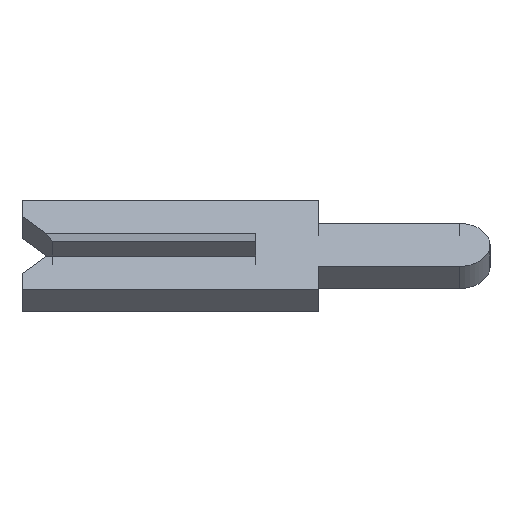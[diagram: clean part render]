
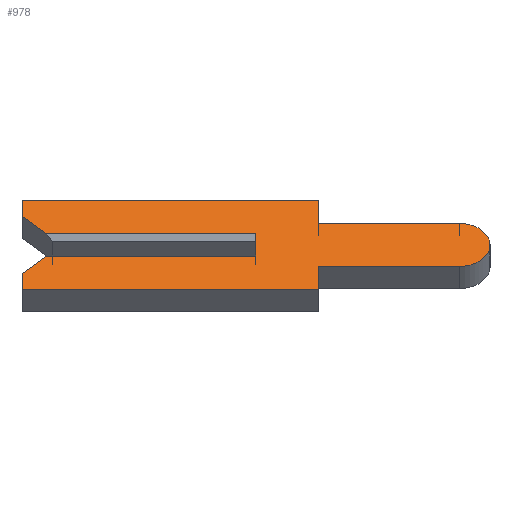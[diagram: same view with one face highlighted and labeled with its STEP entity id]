
A CAD part, left-side view. The second image highlights one B-rep face of the part: STEP entity #978.
In plain terms, the highlighted face is planar.
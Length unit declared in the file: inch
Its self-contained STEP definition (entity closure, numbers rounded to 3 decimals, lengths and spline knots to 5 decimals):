
#20 = CARTESIAN_POINT ( 'NONE',  ( -0.01, -0.04, 0.04 ) ) ;
#44 = LINE ( 'NONE', #263, #1653 ) ;
#54 = ORIENTED_EDGE ( 'NONE', *, *, #1364, .F. ) ;
#75 = CARTESIAN_POINT ( 'NONE',  ( -0.01, -0.1305, 0.0195 ) ) ;
#97 = VECTOR ( 'NONE', #562, 39.37008 ) ;
#116 = VECTOR ( 'NONE', #775, 39.37008 ) ;
#141 = CARTESIAN_POINT ( 'NONE',  ( -0.01, -0.04, -0.04 ) ) ;
#152 = EDGE_CURVE ( 'NONE', #757, #656, #570, .T. ) ;
#189 = ORIENTED_EDGE ( 'NONE', *, *, #524, .F. ) ;
#196 = VERTEX_POINT ( 'NONE', #360 ) ;
#220 = ORIENTED_EDGE ( 'NONE', *, *, #2007, .F. ) ;
#244 = DIRECTION ( 'NONE',  ( 0., 1., 0. ) ) ;
#260 = EDGE_CURVE ( 'NONE', #1860, #1114, #1856, .T. ) ;
#263 = CARTESIAN_POINT ( 'NONE',  ( -0.01, 0., 0.0065 ) ) ;
#295 = DIRECTION ( 'NONE',  ( 0., -0.707, 0.707 ) ) ;
#304 = LINE ( 'NONE', #1445, #460 ) ;
#341 = VECTOR ( 'NONE', #1270, 39.37008 ) ;
#360 = CARTESIAN_POINT ( 'NONE',  ( -0.01, 0.15, 0.026 ) ) ;
#413 = LINE ( 'NONE', #1623, #1289 ) ;
#419 = DIRECTION ( 'NONE',  ( 0., -1., 0. ) ) ;
#432 = CARTESIAN_POINT ( 'NONE',  ( -0.01, 0.134, 0.01 ) ) ;
#441 = CIRCLE ( 'NONE', #1521, 0.0195 ) ;
#446 = CARTESIAN_POINT ( 'NONE',  ( -0.01, -0.04, -0.0195 ) ) ;
#460 = VECTOR ( 'NONE', #1953, 39.37008 ) ;
#491 = LINE ( 'NONE', #798, #1825 ) ;
#512 = VERTEX_POINT ( 'NONE', #1236 ) ;
#517 = LINE ( 'NONE', #1217, #1900 ) ;
#521 = DIRECTION ( 'NONE',  ( 0., 0., -1. ) ) ;
#524 = EDGE_CURVE ( 'NONE', #1607, #1252, #441, .T. ) ;
#562 = DIRECTION ( 'NONE',  ( 0., 0., -1. ) ) ;
#565 = EDGE_CURVE ( 'NONE', #1819, #1348, #682, .T. ) ;
#570 = LINE ( 'NONE', #20, #1478 ) ;
#572 = DIRECTION ( 'NONE',  ( 0., 0., 1. ) ) ;
#584 = LINE ( 'NONE', #907, #2107 ) ;
#595 = EDGE_CURVE ( 'NONE', #196, #905, #517, .T. ) ;
#610 = DIRECTION ( 'NONE',  ( 0., 0., 1. ) ) ;
#618 = CARTESIAN_POINT ( 'NONE',  ( -0.01, 0., -0.01 ) ) ;
#645 = DIRECTION ( 'NONE',  ( 0., -1., 0. ) ) ;
#656 = VERTEX_POINT ( 'NONE', #1936 ) ;
#682 = LINE ( 'NONE', #720, #97 ) ;
#720 = CARTESIAN_POINT ( 'NONE',  ( -0.01, -0.04, -0.04 ) ) ;
#722 = VECTOR ( 'NONE', #419, 39.37008 ) ;
#743 = EDGE_CURVE ( 'NONE', #905, #757, #1164, .T. ) ;
#756 = PLANE ( 'NONE',  #1849 ) ;
#757 = VERTEX_POINT ( 'NONE', #1247 ) ;
#773 = LINE ( 'NONE', #1926, #341 ) ;
#775 = DIRECTION ( 'NONE',  ( 0., 0., 1. ) ) ;
#787 = ORIENTED_EDGE ( 'NONE', *, *, #743, .F. ) ;
#798 = CARTESIAN_POINT ( 'NONE',  ( -0.01, 0.1305, -0.0065 ) ) ;
#838 = VECTOR ( 'NONE', #2056, 39.37008 ) ;
#867 = ORIENTED_EDGE ( 'NONE', *, *, #1035, .F. ) ;
#905 = VERTEX_POINT ( 'NONE', #1113 ) ;
#907 = CARTESIAN_POINT ( 'NONE',  ( -0.01, -0.04, -0.0195 ) ) ;
#908 = VERTEX_POINT ( 'NONE', #618 ) ;
#924 = EDGE_CURVE ( 'NONE', #908, #1114, #44, .T. ) ;
#937 = CARTESIAN_POINT ( 'NONE',  ( -0.01, 0.15, -0.04 ) ) ;
#978 = ADVANCED_FACE ( 'NONE', ( #1962 ), #756, .F. ) ;
#1035 = EDGE_CURVE ( 'NONE', #1935, #908, #773, .T. ) ;
#1049 = DIRECTION ( 'NONE',  ( 1., 0., 0. ) ) ;
#1084 = ORIENTED_EDGE ( 'NONE', *, *, #1249, .F. ) ;
#1113 = CARTESIAN_POINT ( 'NONE',  ( -0.01, 0.15, 0.04 ) ) ;
#1114 = VERTEX_POINT ( 'NONE', #1906 ) ;
#1144 = ORIENTED_EDGE ( 'NONE', *, *, #565, .F. ) ;
#1163 = CARTESIAN_POINT ( 'NONE',  ( -0.01, 0.134, -0.01 ) ) ;
#1164 = LINE ( 'NONE', #1719, #722 ) ;
#1178 = LINE ( 'NONE', #937, #2050 ) ;
#1217 = CARTESIAN_POINT ( 'NONE',  ( -0.01, 0.15, 0.026 ) ) ;
#1236 = CARTESIAN_POINT ( 'NONE',  ( -0.01, 0.15, -0.04 ) ) ;
#1247 = CARTESIAN_POINT ( 'NONE',  ( -0.01, -0.04, 0.04 ) ) ;
#1249 = EDGE_CURVE ( 'NONE', #656, #1607, #413, .T. ) ;
#1252 = VERTEX_POINT ( 'NONE', #1468 ) ;
#1270 = DIRECTION ( 'NONE',  ( 0., -1., 0. ) ) ;
#1289 = VECTOR ( 'NONE', #645, 39.37008 ) ;
#1348 = VERTEX_POINT ( 'NONE', #141 ) ;
#1355 = LINE ( 'NONE', #2095, #116 ) ;
#1364 = EDGE_CURVE ( 'NONE', #1762, #1935, #491, .T. ) ;
#1390 = DIRECTION ( 'NONE',  ( 0., 0., -1. ) ) ;
#1408 = ORIENTED_EDGE ( 'NONE', *, *, #595, .F. ) ;
#1445 = CARTESIAN_POINT ( 'NONE',  ( -0.01, 0.1305, 0.0065 ) ) ;
#1468 = CARTESIAN_POINT ( 'NONE',  ( -0.01, -0.1305, -0.0195 ) ) ;
#1478 = VECTOR ( 'NONE', #521, 39.37008 ) ;
#1503 = ORIENTED_EDGE ( 'NONE', *, *, #1781, .F. ) ;
#1521 = AXIS2_PLACEMENT_3D ( 'NONE', #1709, #1049, #1390 ) ;
#1554 = ORIENTED_EDGE ( 'NONE', *, *, #152, .F. ) ;
#1581 = EDGE_CURVE ( 'NONE', #1252, #1819, #584, .T. ) ;
#1593 = DIRECTION ( 'NONE',  ( 0., 1., 0. ) ) ;
#1607 = VERTEX_POINT ( 'NONE', #75 ) ;
#1623 = CARTESIAN_POINT ( 'NONE',  ( -0.01, -0.04, 0.0195 ) ) ;
#1638 = ORIENTED_EDGE ( 'NONE', *, *, #260, .T. ) ;
#1653 = VECTOR ( 'NONE', #610, 39.37008 ) ;
#1658 = ORIENTED_EDGE ( 'NONE', *, *, #2043, .F. ) ;
#1709 = CARTESIAN_POINT ( 'NONE',  ( -0.01, -0.1305, 0. ) ) ;
#1719 = CARTESIAN_POINT ( 'NONE',  ( -0.01, 0.15, 0.04 ) ) ;
#1757 = CARTESIAN_POINT ( 'NONE',  ( -0.01, -0.1305, 0. ) ) ;
#1762 = VERTEX_POINT ( 'NONE', #1910 ) ;
#1781 = EDGE_CURVE ( 'NONE', #1348, #512, #1178, .T. ) ;
#1819 = VERTEX_POINT ( 'NONE', #446 ) ;
#1825 = VECTOR ( 'NONE', #295, 39.37008 ) ;
#1849 = AXIS2_PLACEMENT_3D ( 'NONE', #1757, #1934, #2070 ) ;
#1856 = LINE ( 'NONE', #2019, #838 ) ;
#1860 = VERTEX_POINT ( 'NONE', #432 ) ;
#1891 = ORIENTED_EDGE ( 'NONE', *, *, #924, .F. ) ;
#1900 = VECTOR ( 'NONE', #572, 39.37008 ) ;
#1906 = CARTESIAN_POINT ( 'NONE',  ( -0.01, 0., 0.01 ) ) ;
#1910 = CARTESIAN_POINT ( 'NONE',  ( -0.01, 0.15, -0.026 ) ) ;
#1926 = CARTESIAN_POINT ( 'NONE',  ( -0.01, -0.1305, -0.01 ) ) ;
#1934 = DIRECTION ( 'NONE',  ( 1., 0., 0. ) ) ;
#1935 = VERTEX_POINT ( 'NONE', #1163 ) ;
#1936 = CARTESIAN_POINT ( 'NONE',  ( -0.01, -0.04, 0.0195 ) ) ;
#1953 = DIRECTION ( 'NONE',  ( 0., 0.707, 0.707 ) ) ;
#1962 = FACE_OUTER_BOUND ( 'NONE', #2097, .T. ) ;
#1968 = ORIENTED_EDGE ( 'NONE', *, *, #1581, .F. ) ;
#2007 = EDGE_CURVE ( 'NONE', #512, #1762, #1355, .T. ) ;
#2019 = CARTESIAN_POINT ( 'NONE',  ( -0.01, 0.15, 0.01 ) ) ;
#2043 = EDGE_CURVE ( 'NONE', #1860, #196, #304, .T. ) ;
#2050 = VECTOR ( 'NONE', #244, 39.37008 ) ;
#2056 = DIRECTION ( 'NONE',  ( 0., -1., 0. ) ) ;
#2070 = DIRECTION ( 'NONE',  ( 0., 0., -1. ) ) ;
#2095 = CARTESIAN_POINT ( 'NONE',  ( -0.01, 0.15, -0.026 ) ) ;
#2097 = EDGE_LOOP ( 'NONE', ( #1638, #1891, #867, #54, #220, #1503, #1144, #1968, #189, #1084, #1554, #787, #1408, #1658 ) ) ;
#2107 = VECTOR ( 'NONE', #1593, 39.37008 ) ;
